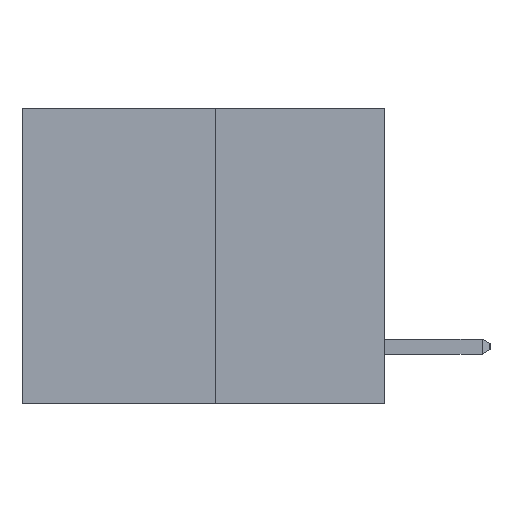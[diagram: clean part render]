
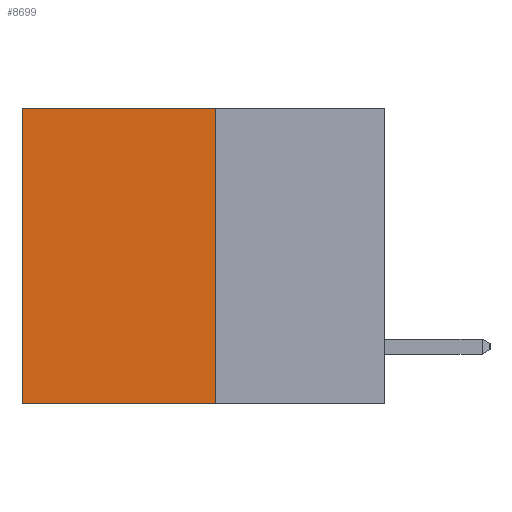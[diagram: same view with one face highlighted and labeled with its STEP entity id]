
A CAD part, left-side view. The second image highlights one B-rep face of the part: STEP entity #8699.
In plain terms, the highlighted planar face has unit normal (-1, 0, 0).
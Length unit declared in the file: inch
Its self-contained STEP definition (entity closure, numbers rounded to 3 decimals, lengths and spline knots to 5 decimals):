
#528 = LINE ( 'NONE', #8796, #9215 ) ;
#854 = LINE ( 'NONE', #6630, #989 ) ;
#989 = VECTOR ( 'NONE', #7538, 39.37008 ) ;
#1048 = CARTESIAN_POINT ( 'NONE',  ( 0.3165, 0.6, 0. ) ) ;
#1314 = DIRECTION ( 'NONE',  ( 0., 0., -1. ) ) ;
#1343 = CARTESIAN_POINT ( 'NONE',  ( 0.3165, 0.28, -0.49 ) ) ;
#1643 = VECTOR ( 'NONE', #5237, 39.37008 ) ;
#3025 = EDGE_CURVE ( 'NONE', #6511, #3405, #854, .T. ) ;
#3405 = VERTEX_POINT ( 'NONE', #4088 ) ;
#3487 = CARTESIAN_POINT ( 'NONE',  ( 0.3165, 0.28, 0. ) ) ;
#3796 = CARTESIAN_POINT ( 'NONE',  ( 0.3165, 0.6, -0.49 ) ) ;
#3972 = CARTESIAN_POINT ( 'NONE',  ( 0.3165, 0.28, 0. ) ) ;
#4088 = CARTESIAN_POINT ( 'NONE',  ( 0.3165, 0.6, -0.49 ) ) ;
#4643 = EDGE_LOOP ( 'NONE', ( #5481, #8516, #10074, #5072 ) ) ;
#4974 = AXIS2_PLACEMENT_3D ( 'NONE', #1343, #10770, #1314 ) ;
#5072 = ORIENTED_EDGE ( 'NONE', *, *, #7311, .T. ) ;
#5237 = DIRECTION ( 'NONE',  ( 0., 1., 0. ) ) ;
#5315 = LINE ( 'NONE', #3487, #1643 ) ;
#5481 = ORIENTED_EDGE ( 'NONE', *, *, #8167, .T. ) ;
#5842 = VECTOR ( 'NONE', #10602, 39.37008 ) ;
#6379 = CARTESIAN_POINT ( 'NONE',  ( 0.3165, 0.28, -0.49 ) ) ;
#6511 = VERTEX_POINT ( 'NONE', #6379 ) ;
#6630 = CARTESIAN_POINT ( 'NONE',  ( 0.3165, 0.28, -0.49 ) ) ;
#7179 = FACE_OUTER_BOUND ( 'NONE', #4643, .T. ) ;
#7311 = EDGE_CURVE ( 'NONE', #10767, #8120, #5315, .T. ) ;
#7538 = DIRECTION ( 'NONE',  ( 0., 1., 0. ) ) ;
#8120 = VERTEX_POINT ( 'NONE', #1048 ) ;
#8167 = EDGE_CURVE ( 'NONE', #8120, #3405, #10333, .T. ) ;
#8303 = PLANE ( 'NONE',  #4974 ) ;
#8516 = ORIENTED_EDGE ( 'NONE', *, *, #3025, .F. ) ;
#8528 = EDGE_CURVE ( 'NONE', #10767, #6511, #528, .T. ) ;
#8699 = ADVANCED_FACE ( 'NONE', ( #7179 ), #8303, .F. ) ;
#8796 = CARTESIAN_POINT ( 'NONE',  ( 0.3165, 0.28, -0.49 ) ) ;
#9215 = VECTOR ( 'NONE', #10551, 39.37008 ) ;
#10074 = ORIENTED_EDGE ( 'NONE', *, *, #8528, .F. ) ;
#10333 = LINE ( 'NONE', #3796, #5842 ) ;
#10551 = DIRECTION ( 'NONE',  ( 0., 0., -1. ) ) ;
#10602 = DIRECTION ( 'NONE',  ( 0., 0., -1. ) ) ;
#10767 = VERTEX_POINT ( 'NONE', #3972 ) ;
#10770 = DIRECTION ( 'NONE',  ( 1., 0., 0. ) ) ;
